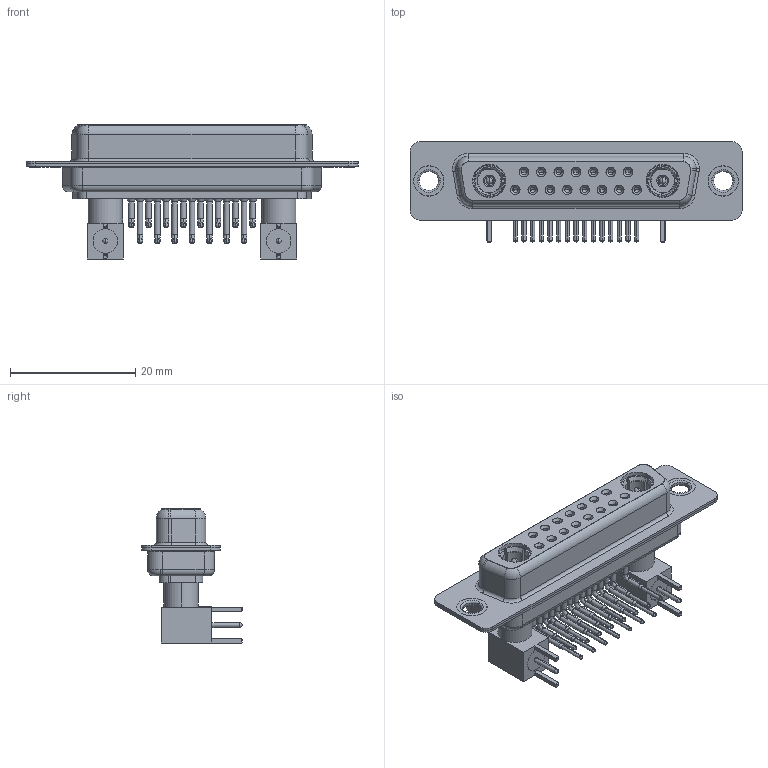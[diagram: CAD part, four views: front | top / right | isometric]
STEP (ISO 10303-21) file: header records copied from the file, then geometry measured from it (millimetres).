
FILE_DESCRIPTION (( 'STEP AP203' ), '1' );
FILE_NAME ('630-17W2640-7N1.STEP', '2022-06-02T16:00:34', ( '' ), ( '' ), 'SwSTEP 2.0', 'SolidWorks 2020', '' );
FILE_SCHEMA (( 'CONFIG_CONTROL_DESIGN' ));
Length unit declared in the file: millimetre
Products named in the file (15): Co-Ax Plug_RA PC Tail; Co-Ax Plug Assy_RA; 630Combo Contact Row 1; 630Combo Housing_17W2; 630-17W2640-7N1; Locking Collar; 630Combo Shell Rear_25 Contacts; Insulator RA Pin; Insulator Pin_Straight PC Tail; 630Combo Shell Front_25 Contacts; Pin_RA; 630Combo Thru Hole Rivet; RA Back Shell; 630Combo Contact Row 2
Assembly tree (34 placements, depth 3):
  630-17W2640-7N1
    630Combo Housing_17W2
    630Combo Shell Front_25 Contacts
    630Combo Shell Rear_25 Contacts
    630Combo Thru Hole Rivet  x2
    Co-Ax Plug Assy_RA
      Co-Ax Plug_RA PC Tail
      Insulator Pin_Straight PC Tail
      Pin_RA
      Locking Collar
      RA Back Shell
      Insulator RA Pin
    Co-Ax Plug Assy_RA
      Co-Ax Plug_RA PC Tail
      Insulator Pin_Straight PC Tail
      Pin_RA
      Locking Collar
      RA Back Shell
      Insulator RA Pin
    630Combo Contact Row 1  x7
    630Combo Contact Row 2  x8
Bounding box: 53.05 x 16 x 21.41 mm (x, y, z)
Volume: 4278.6 mm3; surface area: 10274.6 mm2
Topology: 32 solids, 32 shells, 1384 faces, 3430 edges, 2148 vertices
Faces by surface type: cylinder 596, plane 426, cone 215, torus 77, bspline 62, sphere 8
Entity records: 22400 total; most frequent: CARTESIAN_POINT 3915, DIRECTION 3769, ORIENTED_EDGE 3180, EDGE_CURVE 1590, AXIS2_PLACEMENT_3D 1555, VERTEX_POINT 1008, CIRCLE 844, EDGE_LOOP 812
